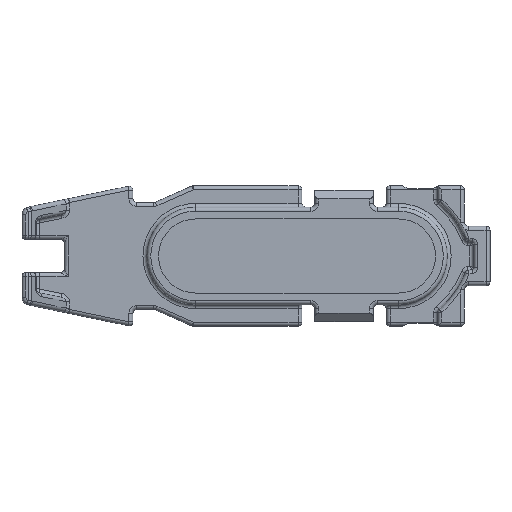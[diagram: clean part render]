
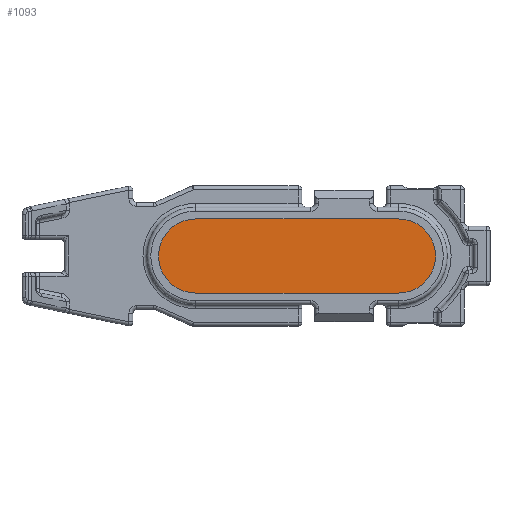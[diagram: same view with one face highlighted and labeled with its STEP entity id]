
A CAD part, front view. The second image highlights one B-rep face of the part: STEP entity #1093.
In plain terms, the highlighted face is planar.
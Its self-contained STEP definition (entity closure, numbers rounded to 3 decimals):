
#18 = DIRECTION ( 'NONE',  ( 0., -1., 0. ) ) ;
#409 = CARTESIAN_POINT ( 'NONE',  ( -7.738, 4.75, 6.1 ) ) ;
#456 = DIRECTION ( 'NONE',  ( 0., 0., 1. ) ) ;
#684 = VERTEX_POINT ( 'NONE', #409 ) ;
#947 = EDGE_CURVE ( 'NONE', #3443, #684, #3955, .T. ) ;
#951 = ORIENTED_EDGE ( 'NONE', *, *, #2105, .T. ) ;
#969 = VERTEX_POINT ( 'NONE', #3213 ) ;
#1093 = ADVANCED_FACE ( 'NONE', ( #2265 ), #6052, .F. ) ;
#1283 = VECTOR ( 'NONE', #4221, 1000. ) ;
#1571 = AXIS2_PLACEMENT_3D ( 'NONE', #7907, #1615, #5309 ) ;
#1615 = DIRECTION ( 'NONE',  ( 0., 0., -1. ) ) ;
#1717 = ORIENTED_EDGE ( 'NONE', *, *, #5063, .T. ) ;
#1974 = ORIENTED_EDGE ( 'NONE', *, *, #2944, .T. ) ;
#2105 = EDGE_CURVE ( 'NONE', #684, #969, #6343, .T. ) ;
#2265 = FACE_OUTER_BOUND ( 'NONE', #2725, .T. ) ;
#2636 = VERTEX_POINT ( 'NONE', #7727 ) ;
#2725 = EDGE_LOOP ( 'NONE', ( #4942, #951, #1717, #1974 ) ) ;
#2769 = AXIS2_PLACEMENT_3D ( 'NONE', #5741, #7645, #18 ) ;
#2905 = CIRCLE ( 'NONE', #2769, 4.75 ) ;
#2944 = EDGE_CURVE ( 'NONE', #2636, #3443, #2905, .T. ) ;
#3213 = CARTESIAN_POINT ( 'NONE',  ( -7.738, -4.75, 6.1 ) ) ;
#3443 = VERTEX_POINT ( 'NONE', #5273 ) ;
#3955 = LINE ( 'NONE', #5157, #5634 ) ;
#4161 = CARTESIAN_POINT ( 'NONE',  ( -7.738, 0., 6.1 ) ) ;
#4221 = DIRECTION ( 'NONE',  ( 1., 0., 0. ) ) ;
#4942 = ORIENTED_EDGE ( 'NONE', *, *, #947, .T. ) ;
#4966 = CARTESIAN_POINT ( 'NONE',  ( -7.738, -4.75, 6.1 ) ) ;
#5021 = AXIS2_PLACEMENT_3D ( 'NONE', #4161, #456, #6684 ) ;
#5063 = EDGE_CURVE ( 'NONE', #969, #2636, #6855, .T. ) ;
#5157 = CARTESIAN_POINT ( 'NONE',  ( -7.738, 4.75, 6.1 ) ) ;
#5273 = CARTESIAN_POINT ( 'NONE',  ( 18.262, 4.75, 6.1 ) ) ;
#5309 = DIRECTION ( 'NONE',  ( 0., 1., 0. ) ) ;
#5634 = VECTOR ( 'NONE', #7557, 1000. ) ;
#5741 = CARTESIAN_POINT ( 'NONE',  ( 18.262, 0., 6.1 ) ) ;
#6052 = PLANE ( 'NONE',  #1571 ) ;
#6343 = CIRCLE ( 'NONE', #5021, 4.75 ) ;
#6684 = DIRECTION ( 'NONE',  ( 0., -1., 0. ) ) ;
#6855 = LINE ( 'NONE', #4966, #1283 ) ;
#7557 = DIRECTION ( 'NONE',  ( -1., 0., 0. ) ) ;
#7645 = DIRECTION ( 'NONE',  ( 0., 0., 1. ) ) ;
#7727 = CARTESIAN_POINT ( 'NONE',  ( 18.262, -4.75, 6.1 ) ) ;
#7907 = CARTESIAN_POINT ( 'NONE',  ( -28.988, 5.286, 6.1 ) ) ;
